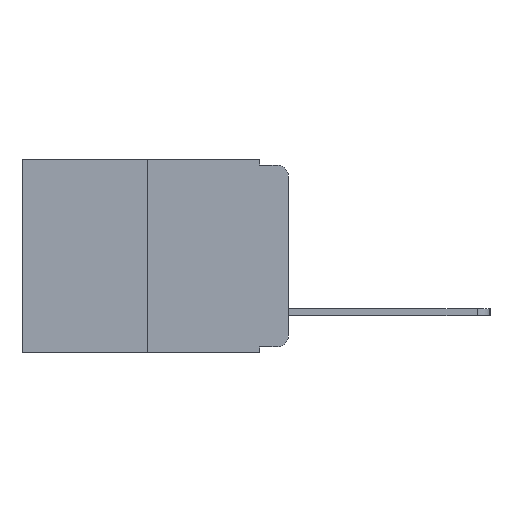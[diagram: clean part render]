
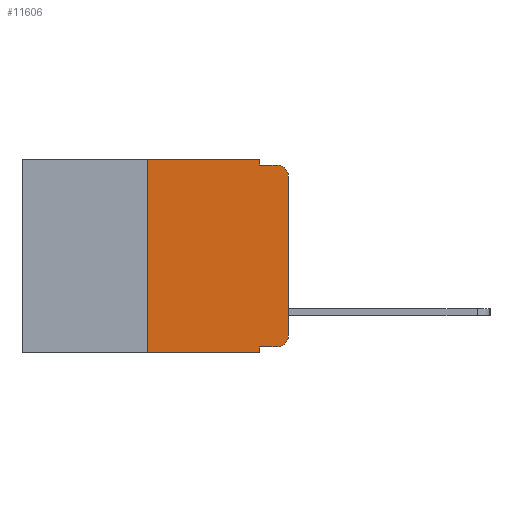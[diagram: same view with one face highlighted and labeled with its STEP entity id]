
A CAD part, left-side view. The second image highlights one B-rep face of the part: STEP entity #11606.
In plain terms, the highlighted planar face has unit normal (-1, 0, 0).
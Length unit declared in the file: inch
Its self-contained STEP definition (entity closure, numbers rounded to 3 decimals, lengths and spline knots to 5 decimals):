
#34 = EDGE_CURVE ( 'NONE', #160, #12864, #7786, .T. ) ;
#67 = VERTEX_POINT ( 'NONE', #2731 ) ;
#160 = VERTEX_POINT ( 'NONE', #12181 ) ;
#187 = VECTOR ( 'NONE', #14016, 39.37008 ) ;
#416 = ORIENTED_EDGE ( 'NONE', *, *, #10625, .F. ) ;
#418 = AXIS2_PLACEMENT_3D ( 'NONE', #3349, #11942, #4646 ) ;
#841 = ORIENTED_EDGE ( 'NONE', *, *, #8227, .F. ) ;
#873 = DIRECTION ( 'NONE',  ( 0., -1., 0. ) ) ;
#986 = AXIS2_PLACEMENT_3D ( 'NONE', #15784, #5052, #13502 ) ;
#1647 = CARTESIAN_POINT ( 'NONE',  ( 0., 0., -0.313 ) ) ;
#1667 = CARTESIAN_POINT ( 'NONE',  ( 0., 0., 0. ) ) ;
#1679 = ORIENTED_EDGE ( 'NONE', *, *, #4022, .T. ) ;
#2266 = EDGE_CURVE ( 'NONE', #4172, #14418, #6960, .T. ) ;
#2731 = CARTESIAN_POINT ( 'NONE',  ( 0., 0.02, -0.01 ) ) ;
#3039 = CARTESIAN_POINT ( 'NONE',  ( 0., 0.051, 0. ) ) ;
#3349 = CARTESIAN_POINT ( 'NONE',  ( 0., 0.02, -0.03 ) ) ;
#3356 = VERTEX_POINT ( 'NONE', #12633 ) ;
#3523 = ORIENTED_EDGE ( 'NONE', *, *, #13826, .T. ) ;
#3708 = LINE ( 'NONE', #1667, #187 ) ;
#3737 = PLANE ( 'NONE',  #986 ) ;
#4010 = VECTOR ( 'NONE', #13760, 39.37008 ) ;
#4022 = EDGE_CURVE ( 'NONE', #4460, #4172, #14031, .T. ) ;
#4172 = VERTEX_POINT ( 'NONE', #8108 ) ;
#4173 = DIRECTION ( 'NONE',  ( 0., 0., -1. ) ) ;
#4278 = DIRECTION ( 'NONE',  ( 0., -1., 0. ) ) ;
#4337 = ORIENTED_EDGE ( 'NONE', *, *, #15917, .F. ) ;
#4441 = VECTOR ( 'NONE', #4577, 39.37008 ) ;
#4460 = VERTEX_POINT ( 'NONE', #5980 ) ;
#4566 = CARTESIAN_POINT ( 'NONE',  ( 0., 0.051, -0.333 ) ) ;
#4577 = DIRECTION ( 'NONE',  ( 0., -1., 0. ) ) ;
#4646 = DIRECTION ( 'NONE',  ( 0., 0., -1. ) ) ;
#4741 = ORIENTED_EDGE ( 'NONE', *, *, #7403, .F. ) ;
#5052 = DIRECTION ( 'NONE',  ( 1., 0., 0. ) ) ;
#5980 = CARTESIAN_POINT ( 'NONE',  ( 0., 0.051, -0.333 ) ) ;
#6123 = VECTOR ( 'NONE', #4278, 39.37008 ) ;
#6240 = LINE ( 'NONE', #9176, #11912 ) ;
#6513 = LINE ( 'NONE', #11610, #6123 ) ;
#6560 = EDGE_CURVE ( 'NONE', #4460, #12864, #6240, .T. ) ;
#6960 = CIRCLE ( 'NONE', #14106, 0.02 ) ;
#7344 = DIRECTION ( 'NONE',  ( 0., 0., 1. ) ) ;
#7403 = EDGE_CURVE ( 'NONE', #160, #13132, #9837, .T. ) ;
#7676 = ORIENTED_EDGE ( 'NONE', *, *, #34, .T. ) ;
#7758 = LINE ( 'NONE', #12529, #4010 ) ;
#7786 = LINE ( 'NONE', #8134, #4441 ) ;
#8108 = CARTESIAN_POINT ( 'NONE',  ( 0., 0.02, -0.333 ) ) ;
#8134 = CARTESIAN_POINT ( 'NONE',  ( 0., 0.473, -0.343 ) ) ;
#8227 = EDGE_CURVE ( 'NONE', #10166, #3356, #7758, .T. ) ;
#8439 = ORIENTED_EDGE ( 'NONE', *, *, #2266, .T. ) ;
#8518 = CARTESIAN_POINT ( 'NONE',  ( 0., 0.473, 0. ) ) ;
#8878 = CARTESIAN_POINT ( 'NONE',  ( 0., 0.25, 0. ) ) ;
#9176 = CARTESIAN_POINT ( 'NONE',  ( 0., 0.051, 0. ) ) ;
#9468 = LINE ( 'NONE', #8518, #15740 ) ;
#9837 = LINE ( 'NONE', #15648, #15744 ) ;
#10166 = VERTEX_POINT ( 'NONE', #3039 ) ;
#10625 = EDGE_CURVE ( 'NONE', #3356, #67, #6513, .T. ) ;
#10706 = DIRECTION ( 'NONE',  ( 0., -1., 0. ) ) ;
#10712 = CARTESIAN_POINT ( 'NONE',  ( 0., 0.051, -0.343 ) ) ;
#10862 = VECTOR ( 'NONE', #10706, 39.37008 ) ;
#11233 = ORIENTED_EDGE ( 'NONE', *, *, #6560, .F. ) ;
#11419 = EDGE_CURVE ( 'NONE', #15197, #67, #14441, .T. ) ;
#11606 = ADVANCED_FACE ( 'NONE', ( #15338 ), #3737, .F. ) ;
#11610 = CARTESIAN_POINT ( 'NONE',  ( 0., 0.051, -0.01 ) ) ;
#11679 = DIRECTION ( 'NONE',  ( -1., 0., 0. ) ) ;
#11877 = CARTESIAN_POINT ( 'NONE',  ( 0., 0., -0.03 ) ) ;
#11912 = VECTOR ( 'NONE', #4173, 39.37008 ) ;
#11942 = DIRECTION ( 'NONE',  ( -1., 0., 0. ) ) ;
#12181 = CARTESIAN_POINT ( 'NONE',  ( 0., 0.25, -0.343 ) ) ;
#12529 = CARTESIAN_POINT ( 'NONE',  ( 0., 0.051, 0. ) ) ;
#12633 = CARTESIAN_POINT ( 'NONE',  ( 0., 0.051, -0.01 ) ) ;
#12864 = VERTEX_POINT ( 'NONE', #10712 ) ;
#13132 = VERTEX_POINT ( 'NONE', #8878 ) ;
#13184 = EDGE_LOOP ( 'NONE', ( #3523, #13274, #416, #841, #4337, #4741, #7676, #11233, #1679, #8439 ) ) ;
#13274 = ORIENTED_EDGE ( 'NONE', *, *, #11419, .T. ) ;
#13502 = DIRECTION ( 'NONE',  ( 0., 0., -1. ) ) ;
#13760 = DIRECTION ( 'NONE',  ( 0., 0., -1. ) ) ;
#13826 = EDGE_CURVE ( 'NONE', #14418, #15197, #3708, .T. ) ;
#14016 = DIRECTION ( 'NONE',  ( 0., 0., 1. ) ) ;
#14031 = LINE ( 'NONE', #4566, #10862 ) ;
#14106 = AXIS2_PLACEMENT_3D ( 'NONE', #15033, #11679, #14320 ) ;
#14320 = DIRECTION ( 'NONE',  ( 0., 0., -1. ) ) ;
#14418 = VERTEX_POINT ( 'NONE', #1647 ) ;
#14441 = CIRCLE ( 'NONE', #418, 0.02 ) ;
#15033 = CARTESIAN_POINT ( 'NONE',  ( 0., 0.02, -0.313 ) ) ;
#15197 = VERTEX_POINT ( 'NONE', #11877 ) ;
#15338 = FACE_OUTER_BOUND ( 'NONE', #13184, .T. ) ;
#15648 = CARTESIAN_POINT ( 'NONE',  ( 0., 0.25, 0. ) ) ;
#15740 = VECTOR ( 'NONE', #873, 39.37008 ) ;
#15744 = VECTOR ( 'NONE', #7344, 39.37008 ) ;
#15784 = CARTESIAN_POINT ( 'NONE',  ( 0., 0.473, 0. ) ) ;
#15917 = EDGE_CURVE ( 'NONE', #13132, #10166, #9468, .T. ) ;
